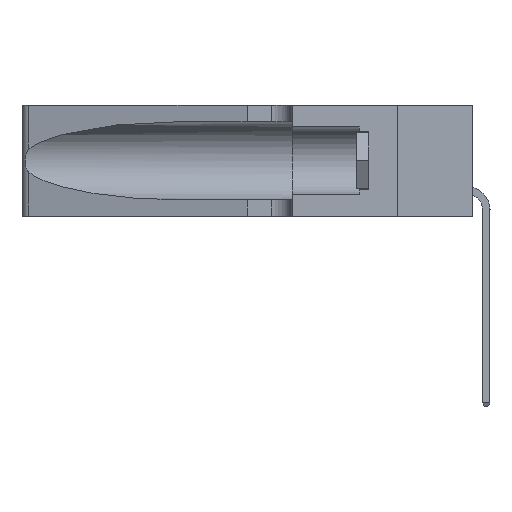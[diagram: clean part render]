
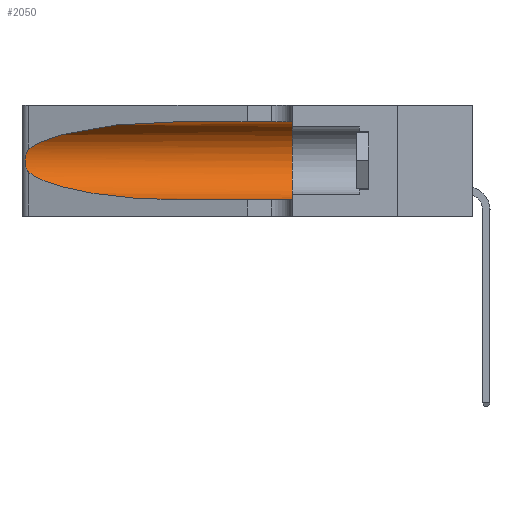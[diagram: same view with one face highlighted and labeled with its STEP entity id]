
A CAD part, left-side view. The second image highlights one B-rep face of the part: STEP entity #2050.
In plain terms, the highlighted cylindrical face has radius 3.308 mm (diameter 6.617 mm), a partial arc.
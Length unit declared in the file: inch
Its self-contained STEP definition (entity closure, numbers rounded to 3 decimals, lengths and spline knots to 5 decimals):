
#168 = LINE ( 'NONE', #16210, #4604 ) ;
#227 = CARTESIAN_POINT ( 'NONE',  ( 0.1305, 0.72297, 0.05475 ) ) ;
#543 = AXIS2_PLACEMENT_3D ( 'NONE', #2556, #12719, #7614 ) ;
#1361 = CARTESIAN_POINT ( 'NONE',  ( 0.2373, 1.15595, 0.08982 ) ) ;
#1695 = VERTEX_POINT ( 'NONE', #4361 ) ;
#1914 = CARTESIAN_POINT ( 'NONE',  ( 0.2373, 1.15595, 0.28018 ) ) ;
#1949 = ORIENTED_EDGE ( 'NONE', *, *, #5934, .T. ) ;
#2050 = ADVANCED_FACE ( 'NONE', ( #6641 ), #11232, .F. ) ;
#2142 = VERTEX_POINT ( 'NONE', #13114 ) ;
#2556 = CARTESIAN_POINT ( 'NONE',  ( 0.1305, 1.61858, 0.185 ) ) ;
#2774 = CARTESIAN_POINT ( 'NONE',  ( 0.18966, 0.96281, 0.05475 ) ) ;
#3022 = LINE ( 'NONE', #3566, #9383 ) ;
#3435 = DIRECTION ( 'NONE',  ( 0., -1., 0. ) ) ;
#3566 = CARTESIAN_POINT ( 'NONE',  ( 0.1305, 1.61858, 0.05475 ) ) ;
#4072 = EDGE_CURVE ( 'NONE', #10332, #2142, #6123, .T. ) ;
#4361 = CARTESIAN_POINT ( 'NONE',  ( 0.1305, 0.35, 0.05475 ) ) ;
#4499 = CARTESIAN_POINT ( 'NONE',  ( 0.25487, 1.22718, 0.22369 ) ) ;
#4541 = VERTEX_POINT ( 'NONE', #13999 ) ;
#4543 = CARTESIAN_POINT ( 'NONE',  ( 0.25787, 1.23484, 0.2124 ) ) ;
#4604 = VECTOR ( 'NONE', #3435, 39.37008 ) ;
#4822 = EDGE_CURVE ( 'NONE', #15107, #1695, #14785, .T. ) ;
#5148 = CARTESIAN_POINT ( 'NONE',  ( 0.26075, 1.23896, 0.178 ) ) ;
#5190 = ORIENTED_EDGE ( 'NONE', *, *, #4822, .F. ) ;
#5251 = CARTESIAN_POINT ( 'NONE',  ( 0.25487, 1.22718, 0.14631 ) ) ;
#5505 = CARTESIAN_POINT ( 'NONE',  ( 0.1305, 0.35, 0.185 ) ) ;
#5776 = CARTESIAN_POINT ( 'NONE',  ( 0.25854, 1.2359, 0.20912 ) ) ;
#5934 = EDGE_CURVE ( 'NONE', #4541, #10332, #6852, .T. ) ;
#6123 =( BOUNDED_CURVE ( )  B_SPLINE_CURVE ( 3, ( #15497, #1361, #2774, #227 ),
 .UNSPECIFIED., .F., .T. ) 
 B_SPLINE_CURVE_WITH_KNOTS ( ( 4, 4 ),
 ( 3.44316, 4.71239 ),
 .UNSPECIFIED. ) 
 CURVE ( )  GEOMETRIC_REPRESENTATION_ITEM ( )  RATIONAL_B_SPLINE_CURVE ( ( 1., 0.87, 0.87, 1. ) ) 
 REPRESENTATION_ITEM ( '' )  );
#6641 = FACE_OUTER_BOUND ( 'NONE', #7965, .T. ) ;
#6835 = DIRECTION ( 'NONE',  ( 0., 0., 1. ) ) ;
#6852 = B_SPLINE_CURVE_WITH_KNOTS ( 'NONE', 3,
 ( #12181, #10708, #10820, #4543, #5776, #11951, #12008, #5148, #12903, #7687, #15291, #7794, #10371, #11672 ),
 .UNSPECIFIED., .F., .F.,
 ( 4, 2, 2, 2, 2, 2, 4 ),
 ( 0., 0.00027, 0.00053, 0.00107, 0.0016, 0.00187, 0.00214 ),
 .UNSPECIFIED. ) ;
#7176 = EDGE_CURVE ( 'NONE', #8080, #4541, #12782, .T. ) ;
#7614 = DIRECTION ( 'NONE',  ( 0., 0., -1. ) ) ;
#7687 = CARTESIAN_POINT ( 'NONE',  ( 0.25856, 1.23593, 0.16098 ) ) ;
#7794 = CARTESIAN_POINT ( 'NONE',  ( 0.25639, 1.23186, 0.15144 ) ) ;
#7965 = EDGE_LOOP ( 'NONE', ( #15491, #1949, #10271, #11278, #5190, #16541 ) ) ;
#8080 = VERTEX_POINT ( 'NONE', #8271 ) ;
#8271 = CARTESIAN_POINT ( 'NONE',  ( 0.1305, 0.72297, 0.31525 ) ) ;
#9383 = VECTOR ( 'NONE', #13826, 39.37008 ) ;
#10271 = ORIENTED_EDGE ( 'NONE', *, *, #4072, .T. ) ;
#10332 = VERTEX_POINT ( 'NONE', #5251 ) ;
#10371 = CARTESIAN_POINT ( 'NONE',  ( 0.25555, 1.22993, 0.14849 ) ) ;
#10708 = CARTESIAN_POINT ( 'NONE',  ( 0.25555, 1.22994, 0.2215 ) ) ;
#10820 = CARTESIAN_POINT ( 'NONE',  ( 0.25639, 1.23184, 0.21858 ) ) ;
#11232 = CYLINDRICAL_SURFACE ( 'NONE', #543, 0.13025 ) ;
#11278 = ORIENTED_EDGE ( 'NONE', *, *, #15384, .T. ) ;
#11672 = CARTESIAN_POINT ( 'NONE',  ( 0.25487, 1.22718, 0.14631 ) ) ;
#11685 = CARTESIAN_POINT ( 'NONE',  ( 0.18966, 0.96281, 0.31525 ) ) ;
#11852 = EDGE_CURVE ( 'NONE', #8080, #15107, #168, .T. ) ;
#11951 = CARTESIAN_POINT ( 'NONE',  ( 0.26018, 1.23835, 0.19895 ) ) ;
#12008 = CARTESIAN_POINT ( 'NONE',  ( 0.26075, 1.23896, 0.19203 ) ) ;
#12181 = CARTESIAN_POINT ( 'NONE',  ( 0.25487, 1.22718, 0.22369 ) ) ;
#12432 = CARTESIAN_POINT ( 'NONE',  ( 0.1305, 0.35, 0.31525 ) ) ;
#12719 = DIRECTION ( 'NONE',  ( 0., -1., 0. ) ) ;
#12782 =( BOUNDED_CURVE ( )  B_SPLINE_CURVE ( 3, ( #14370, #11685, #1914, #4499 ),
 .UNSPECIFIED., .F., .F. ) 
 B_SPLINE_CURVE_WITH_KNOTS ( ( 4, 4 ),
 ( 1.5708, 2.84003 ),
 .UNSPECIFIED. ) 
 CURVE ( )  GEOMETRIC_REPRESENTATION_ITEM ( )  RATIONAL_B_SPLINE_CURVE ( ( 1., 0.87, 0.87, 1. ) ) 
 REPRESENTATION_ITEM ( '' )  );
#12903 = CARTESIAN_POINT ( 'NONE',  ( 0.26017, 1.23833, 0.17102 ) ) ;
#13109 = DIRECTION ( 'NONE',  ( 0., 1., 0. ) ) ;
#13114 = CARTESIAN_POINT ( 'NONE',  ( 0.1305, 0.72297, 0.05475 ) ) ;
#13826 = DIRECTION ( 'NONE',  ( 0., -1., 0. ) ) ;
#13999 = CARTESIAN_POINT ( 'NONE',  ( 0.25487, 1.22718, 0.22369 ) ) ;
#14370 = CARTESIAN_POINT ( 'NONE',  ( 0.1305, 0.72297, 0.31525 ) ) ;
#14785 = CIRCLE ( 'NONE', #16004, 0.13025 ) ;
#15107 = VERTEX_POINT ( 'NONE', #12432 ) ;
#15291 = CARTESIAN_POINT ( 'NONE',  ( 0.25789, 1.23486, 0.15765 ) ) ;
#15384 = EDGE_CURVE ( 'NONE', #2142, #1695, #3022, .T. ) ;
#15491 = ORIENTED_EDGE ( 'NONE', *, *, #7176, .T. ) ;
#15497 = CARTESIAN_POINT ( 'NONE',  ( 0.25487, 1.22718, 0.14631 ) ) ;
#16004 = AXIS2_PLACEMENT_3D ( 'NONE', #5505, #13109, #6835 ) ;
#16210 = CARTESIAN_POINT ( 'NONE',  ( 0.1305, 1.61858, 0.31525 ) ) ;
#16541 = ORIENTED_EDGE ( 'NONE', *, *, #11852, .F. ) ;
